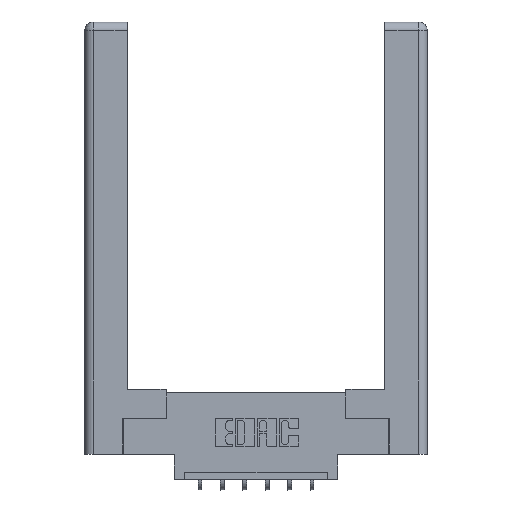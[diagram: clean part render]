
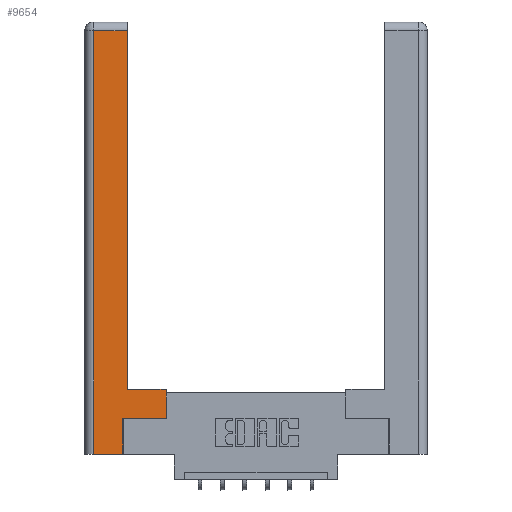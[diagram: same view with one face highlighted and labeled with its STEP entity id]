
A CAD part, top view. The second image highlights one B-rep face of the part: STEP entity #9654.
In plain terms, the highlighted planar face has unit normal (0, 0, 1).
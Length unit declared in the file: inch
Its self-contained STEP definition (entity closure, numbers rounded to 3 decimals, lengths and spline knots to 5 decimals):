
#151 = CARTESIAN_POINT ( 'NONE',  ( 0.0615, 2.94, 0. ) ) ;
#388 = DIRECTION ( 'NONE',  ( 0., 1., 0. ) ) ;
#578 = LINE ( 'NONE', #4388, #9691 ) ;
#664 = VECTOR ( 'NONE', #10412, 39.37008 ) ;
#732 = ORIENTED_EDGE ( 'NONE', *, *, #9067, .T. ) ;
#842 = LINE ( 'NONE', #7854, #5459 ) ;
#908 = LINE ( 'NONE', #11502, #8878 ) ;
#1056 = CARTESIAN_POINT ( 'NONE',  ( 0.295, 0.45, 0. ) ) ;
#1296 = PLANE ( 'NONE',  #1379 ) ;
#1379 = AXIS2_PLACEMENT_3D ( 'NONE', #4004, #11488, #5834 ) ;
#1464 = VECTOR ( 'NONE', #4825, 39.37008 ) ;
#1545 = CARTESIAN_POINT ( 'NONE',  ( 0.295, 2.94, 0. ) ) ;
#1764 = CARTESIAN_POINT ( 'NONE',  ( 0.265, 0., 0. ) ) ;
#1844 = LINE ( 'NONE', #4107, #8949 ) ;
#2591 = VERTEX_POINT ( 'NONE', #1545 ) ;
#2697 = CARTESIAN_POINT ( 'NONE',  ( 0.0615, 2.94, 0. ) ) ;
#3074 = EDGE_CURVE ( 'NONE', #2591, #8056, #3475, .T. ) ;
#3407 = LINE ( 'NONE', #5880, #664 ) ;
#3475 = LINE ( 'NONE', #151, #8980 ) ;
#3591 = DIRECTION ( 'NONE',  ( 1., 0., 0. ) ) ;
#3607 = VERTEX_POINT ( 'NONE', #11220 ) ;
#3832 = EDGE_CURVE ( 'NONE', #3607, #5831, #1844, .T. ) ;
#3974 = VERTEX_POINT ( 'NONE', #7038 ) ;
#4004 = CARTESIAN_POINT ( 'NONE',  ( 0., 0., 0. ) ) ;
#4107 = CARTESIAN_POINT ( 'NONE',  ( 0.565, 0.45, 0. ) ) ;
#4138 = VERTEX_POINT ( 'NONE', #1764 ) ;
#4388 = CARTESIAN_POINT ( 'NONE',  ( 0.265, 0., 0. ) ) ;
#4825 = DIRECTION ( 'NONE',  ( 0., -1., 0. ) ) ;
#4956 = EDGE_LOOP ( 'NONE', ( #732, #11301, #10592, #7877, #6442, #5704, #5006, #7782 ) ) ;
#4991 = VERTEX_POINT ( 'NONE', #7743 ) ;
#5006 = ORIENTED_EDGE ( 'NONE', *, *, #3832, .T. ) ;
#5459 = VECTOR ( 'NONE', #8619, 39.37008 ) ;
#5704 = ORIENTED_EDGE ( 'NONE', *, *, #7136, .T. ) ;
#5831 = VERTEX_POINT ( 'NONE', #7082 ) ;
#5834 = DIRECTION ( 'NONE',  ( -1., 0., 0. ) ) ;
#5880 = CARTESIAN_POINT ( 'NONE',  ( 0.565, 0.245, 0. ) ) ;
#6213 = DIRECTION ( 'NONE',  ( 0., 1., 0. ) ) ;
#6442 = ORIENTED_EDGE ( 'NONE', *, *, #8634, .T. ) ;
#7038 = CARTESIAN_POINT ( 'NONE',  ( 0.265, 0.245, 0. ) ) ;
#7082 = CARTESIAN_POINT ( 'NONE',  ( 0.565, 0.45, 0. ) ) ;
#7136 = EDGE_CURVE ( 'NONE', #3974, #3607, #3407, .T. ) ;
#7743 = CARTESIAN_POINT ( 'NONE',  ( 0.0615, 0., 0. ) ) ;
#7782 = ORIENTED_EDGE ( 'NONE', *, *, #10288, .T. ) ;
#7854 = CARTESIAN_POINT ( 'NONE',  ( 0.295, 0.45, 0. ) ) ;
#7877 = ORIENTED_EDGE ( 'NONE', *, *, #10563, .T. ) ;
#8056 = VERTEX_POINT ( 'NONE', #2697 ) ;
#8457 = LINE ( 'NONE', #9649, #11483 ) ;
#8619 = DIRECTION ( 'NONE',  ( -1., 0., 0. ) ) ;
#8634 = EDGE_CURVE ( 'NONE', #4138, #3974, #8457, .T. ) ;
#8878 = VECTOR ( 'NONE', #388, 39.37008 ) ;
#8949 = VECTOR ( 'NONE', #9708, 39.37008 ) ;
#8980 = VECTOR ( 'NONE', #10399, 39.37008 ) ;
#9067 = EDGE_CURVE ( 'NONE', #11791, #2591, #908, .T. ) ;
#9304 = FACE_OUTER_BOUND ( 'NONE', #4956, .T. ) ;
#9546 = EDGE_CURVE ( 'NONE', #8056, #4991, #10003, .T. ) ;
#9649 = CARTESIAN_POINT ( 'NONE',  ( 0.265, 0.245, 0. ) ) ;
#9654 = ADVANCED_FACE ( 'NONE', ( #9304 ), #1296, .F. ) ;
#9691 = VECTOR ( 'NONE', #3591, 39.37008 ) ;
#9708 = DIRECTION ( 'NONE',  ( 0., 1., 0. ) ) ;
#10003 = LINE ( 'NONE', #10358, #1464 ) ;
#10288 = EDGE_CURVE ( 'NONE', #5831, #11791, #842, .T. ) ;
#10358 = CARTESIAN_POINT ( 'NONE',  ( 0.0615, 0., 0. ) ) ;
#10399 = DIRECTION ( 'NONE',  ( -1., 0., 0. ) ) ;
#10412 = DIRECTION ( 'NONE',  ( 1., 0., 0. ) ) ;
#10563 = EDGE_CURVE ( 'NONE', #4991, #4138, #578, .T. ) ;
#10592 = ORIENTED_EDGE ( 'NONE', *, *, #9546, .T. ) ;
#11220 = CARTESIAN_POINT ( 'NONE',  ( 0.565, 0.245, 0. ) ) ;
#11301 = ORIENTED_EDGE ( 'NONE', *, *, #3074, .T. ) ;
#11483 = VECTOR ( 'NONE', #6213, 39.37008 ) ;
#11488 = DIRECTION ( 'NONE',  ( 0., 0., -1. ) ) ;
#11502 = CARTESIAN_POINT ( 'NONE',  ( 0.295, 3., 0. ) ) ;
#11791 = VERTEX_POINT ( 'NONE', #1056 ) ;
